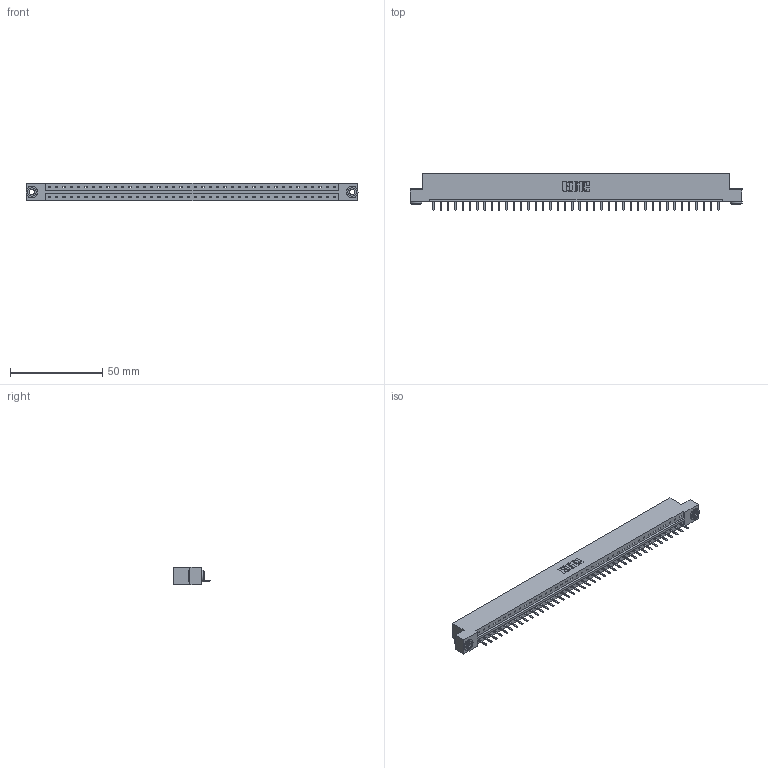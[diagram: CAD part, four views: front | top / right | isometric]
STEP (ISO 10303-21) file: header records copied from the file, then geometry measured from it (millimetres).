
FILE_DESCRIPTION (( 'STEP AP203' ), '1' );
FILE_NAME ('833-040-520-103.STEP', '2020-06-03T15:44:21', ( '' ), ( '' ), 'SwSTEP 2.0', 'SolidWorks 2020', '' );
FILE_SCHEMA (( 'CONFIG_CONTROL_DESIGN' ));
Length unit declared in the file: inch
Products named in the file (4): 345-292-001_345-293-120; 833-040-520-103; 345-250-002_345-250-002-102; 833 Part_Flush - .156 Dia - TH
Assembly tree (43 placements, depth 2):
  833-040-520-103
    833 Part_Flush - .156 Dia - TH
    345-292-001_345-293-120  x40
    345-250-002_345-250-002-102  x2
Bounding box: 180.04 x 20.02 x 9.4 mm (x, y, z)
Volume: 18003.7 mm3; surface area: 19290.6 mm2
Topology: 43 solids, 43 shells, 2632 faces, 7747 edges, 5054 vertices
Faces by surface type: plane 1840, cylinder 784, cone 8
Entity records: 25476 total; most frequent: CARTESIAN_POINT 4385, ORIENTED_EDGE 4342, DIRECTION 3725, EDGE_CURVE 2171, LINE 2015, VECTOR 2015, VERTEX_POINT 1442, AXIS2_PLACEMENT_3D 855
